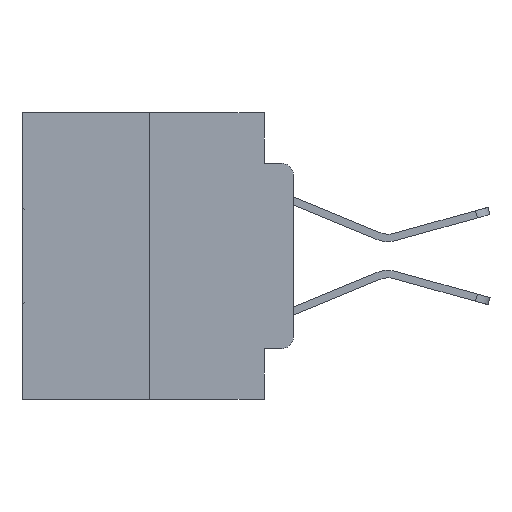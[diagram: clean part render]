
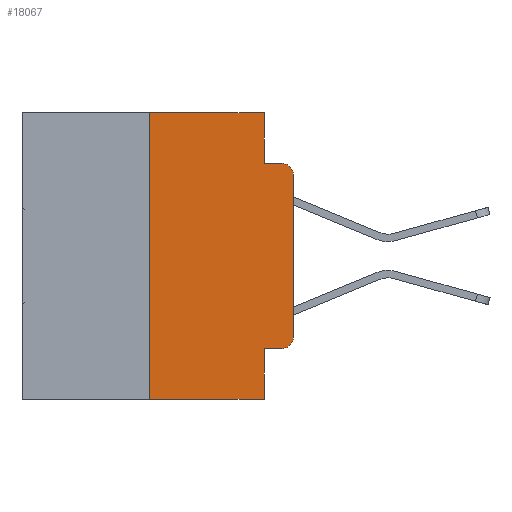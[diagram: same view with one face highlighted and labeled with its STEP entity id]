
A CAD part, left-side view. The second image highlights one B-rep face of the part: STEP entity #18067.
In plain terms, the highlighted planar face has unit normal (-1, 0, 0).
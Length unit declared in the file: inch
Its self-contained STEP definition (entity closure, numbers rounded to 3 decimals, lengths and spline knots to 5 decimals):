
#738 = ORIENTED_EDGE ( 'NONE', *, *, #29867, .F. ) ;
#795 = CIRCLE ( 'NONE', #9008, 0.02 ) ;
#811 = CARTESIAN_POINT ( 'NONE',  ( 0., 0.473, -0.5 ) ) ;
#916 = DIRECTION ( 'NONE',  ( 1., 0., 0. ) ) ;
#923 = EDGE_CURVE ( 'NONE', #1005, #1338, #13358, .T. ) ;
#961 = LINE ( 'NONE', #811, #29965 ) ;
#1005 = VERTEX_POINT ( 'NONE', #4815 ) ;
#1303 = DIRECTION ( 'NONE',  ( 0., 0., -1. ) ) ;
#1338 = VERTEX_POINT ( 'NONE', #28597 ) ;
#1752 = ORIENTED_EDGE ( 'NONE', *, *, #5533, .T. ) ;
#1765 = CARTESIAN_POINT ( 'NONE',  ( 0., 0.051, -0.4115 ) ) ;
#2103 = CARTESIAN_POINT ( 'NONE',  ( 0., 0.051, 0. ) ) ;
#2200 = VECTOR ( 'NONE', #26437, 39.37008 ) ;
#3134 = AXIS2_PLACEMENT_3D ( 'NONE', #30714, #27996, #20746 ) ;
#3643 = LINE ( 'NONE', #28104, #10400 ) ;
#3663 = CIRCLE ( 'NONE', #3134, 0.02 ) ;
#3760 = VECTOR ( 'NONE', #7057, 39.37008 ) ;
#4428 = EDGE_CURVE ( 'NONE', #15823, #6950, #11917, .T. ) ;
#4815 = CARTESIAN_POINT ( 'NONE',  ( 0., 0.25, -0.5 ) ) ;
#5085 = CARTESIAN_POINT ( 'NONE',  ( 0., 0., -0.1085 ) ) ;
#5533 = EDGE_CURVE ( 'NONE', #6272, #6673, #29805, .T. ) ;
#5673 = DIRECTION ( 'NONE',  ( 0., -1., 0. ) ) ;
#6091 = EDGE_CURVE ( 'NONE', #14204, #7328, #3663, .T. ) ;
#6102 = VECTOR ( 'NONE', #28806, 39.37008 ) ;
#6272 = VERTEX_POINT ( 'NONE', #1765 ) ;
#6673 = VERTEX_POINT ( 'NONE', #10047 ) ;
#6950 = VERTEX_POINT ( 'NONE', #16446 ) ;
#6990 = ORIENTED_EDGE ( 'NONE', *, *, #27029, .T. ) ;
#7057 = DIRECTION ( 'NONE',  ( 0., -1., 0. ) ) ;
#7211 = LINE ( 'NONE', #22486, #3760 ) ;
#7328 = VERTEX_POINT ( 'NONE', #20755 ) ;
#7766 = VERTEX_POINT ( 'NONE', #30971 ) ;
#8011 = LINE ( 'NONE', #27302, #19005 ) ;
#8814 = AXIS2_PLACEMENT_3D ( 'NONE', #22467, #916, #30498 ) ;
#9008 = AXIS2_PLACEMENT_3D ( 'NONE', #28303, #13518, #1303 ) ;
#10047 = CARTESIAN_POINT ( 'NONE',  ( 0., 0.02, -0.4115 ) ) ;
#10242 = PLANE ( 'NONE',  #8814 ) ;
#10400 = VECTOR ( 'NONE', #25208, 39.37008 ) ;
#11917 = LINE ( 'NONE', #2103, #6102 ) ;
#12571 = EDGE_CURVE ( 'NONE', #1338, #15823, #8011, .T. ) ;
#12769 = ORIENTED_EDGE ( 'NONE', *, *, #23728, .T. ) ;
#13358 = LINE ( 'NONE', #18824, #29048 ) ;
#13518 = DIRECTION ( 'NONE',  ( -1., 0., 0. ) ) ;
#14204 = VERTEX_POINT ( 'NONE', #5085 ) ;
#14222 = LINE ( 'NONE', #29153, #2200 ) ;
#14722 = ORIENTED_EDGE ( 'NONE', *, *, #12571, .F. ) ;
#15625 = ORIENTED_EDGE ( 'NONE', *, *, #6091, .T. ) ;
#15823 = VERTEX_POINT ( 'NONE', #22460 ) ;
#15955 = VECTOR ( 'NONE', #5673, 39.37008 ) ;
#16097 = VERTEX_POINT ( 'NONE', #17289 ) ;
#16446 = CARTESIAN_POINT ( 'NONE',  ( 0., 0.051, -0.0885 ) ) ;
#17289 = CARTESIAN_POINT ( 'NONE',  ( 0., 0., -0.3915 ) ) ;
#17542 = ORIENTED_EDGE ( 'NONE', *, *, #22970, .T. ) ;
#17579 = CARTESIAN_POINT ( 'NONE',  ( 0., 0.051, -0.4115 ) ) ;
#18067 = ADVANCED_FACE ( 'NONE', ( #20519 ), #10242, .F. ) ;
#18824 = CARTESIAN_POINT ( 'NONE',  ( 0., 0.25, 0. ) ) ;
#19005 = VECTOR ( 'NONE', #30349, 39.37008 ) ;
#20519 = FACE_OUTER_BOUND ( 'NONE', #22466, .T. ) ;
#20746 = DIRECTION ( 'NONE',  ( 0., 0., -1. ) ) ;
#20755 = CARTESIAN_POINT ( 'NONE',  ( 0., 0.02, -0.0885 ) ) ;
#22460 = CARTESIAN_POINT ( 'NONE',  ( 0., 0.051, 0. ) ) ;
#22466 = EDGE_LOOP ( 'NONE', ( #17542, #15625, #738, #23811, #14722, #30782, #12769, #27124, #1752, #6990 ) ) ;
#22467 = CARTESIAN_POINT ( 'NONE',  ( 0., 0.473, 0. ) ) ;
#22486 = CARTESIAN_POINT ( 'NONE',  ( 0., 0.051, -0.0885 ) ) ;
#22970 = EDGE_CURVE ( 'NONE', #16097, #14204, #14222, .T. ) ;
#23728 = EDGE_CURVE ( 'NONE', #1005, #7766, #961, .T. ) ;
#23811 = ORIENTED_EDGE ( 'NONE', *, *, #4428, .F. ) ;
#24165 = EDGE_CURVE ( 'NONE', #6272, #7766, #3643, .T. ) ;
#25208 = DIRECTION ( 'NONE',  ( 0., 0., -1. ) ) ;
#26437 = DIRECTION ( 'NONE',  ( 0., 0., 1. ) ) ;
#27029 = EDGE_CURVE ( 'NONE', #6673, #16097, #795, .T. ) ;
#27124 = ORIENTED_EDGE ( 'NONE', *, *, #24165, .F. ) ;
#27302 = CARTESIAN_POINT ( 'NONE',  ( 0., 0.473, 0. ) ) ;
#27996 = DIRECTION ( 'NONE',  ( -1., 0., 0. ) ) ;
#28104 = CARTESIAN_POINT ( 'NONE',  ( 0., 0.051, 0. ) ) ;
#28303 = CARTESIAN_POINT ( 'NONE',  ( 0., 0.02, -0.3915 ) ) ;
#28597 = CARTESIAN_POINT ( 'NONE',  ( 0., 0.25, 0. ) ) ;
#28806 = DIRECTION ( 'NONE',  ( 0., 0., -1. ) ) ;
#29048 = VECTOR ( 'NONE', #30572, 39.37008 ) ;
#29153 = CARTESIAN_POINT ( 'NONE',  ( 0., 0., 0. ) ) ;
#29805 = LINE ( 'NONE', #17579, #15955 ) ;
#29867 = EDGE_CURVE ( 'NONE', #6950, #7328, #7211, .T. ) ;
#29965 = VECTOR ( 'NONE', #30226, 39.37008 ) ;
#30226 = DIRECTION ( 'NONE',  ( 0., -1., 0. ) ) ;
#30349 = DIRECTION ( 'NONE',  ( 0., -1., 0. ) ) ;
#30498 = DIRECTION ( 'NONE',  ( 0., 0., -1. ) ) ;
#30572 = DIRECTION ( 'NONE',  ( 0., 0., 1. ) ) ;
#30714 = CARTESIAN_POINT ( 'NONE',  ( 0., 0.02, -0.1085 ) ) ;
#30782 = ORIENTED_EDGE ( 'NONE', *, *, #923, .F. ) ;
#30971 = CARTESIAN_POINT ( 'NONE',  ( 0., 0.051, -0.5 ) ) ;
